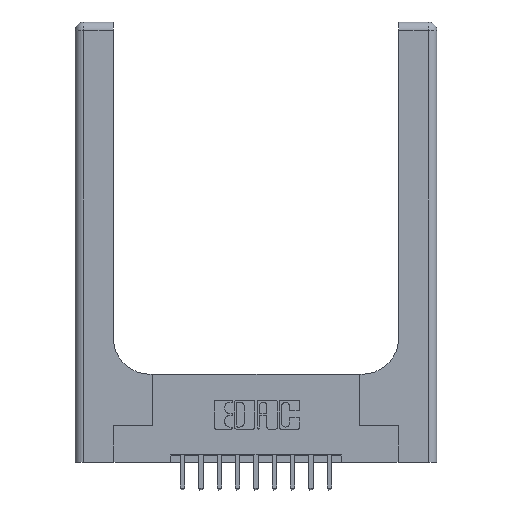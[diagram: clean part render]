
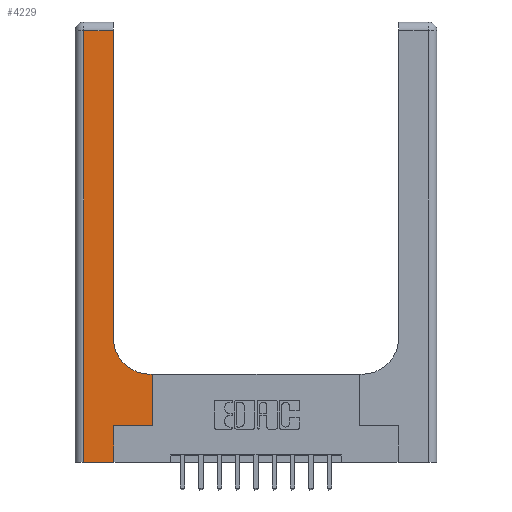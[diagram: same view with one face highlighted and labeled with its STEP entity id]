
A CAD part, top view. The second image highlights one B-rep face of the part: STEP entity #4229.
In plain terms, the highlighted planar face has unit normal (0, 0, 1).
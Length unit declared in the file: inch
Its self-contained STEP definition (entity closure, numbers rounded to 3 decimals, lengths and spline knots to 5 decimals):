
#92 = DIRECTION ( 'NONE',  ( 1., 0., 0. ) ) ;
#148 = CARTESIAN_POINT ( 'NONE',  ( 0.51, 0.85, 0.37 ) ) ;
#991 = VECTOR ( 'NONE', #5876, 39.37008 ) ;
#1242 = EDGE_CURVE ( 'NONE', #6423, #10171, #7433, .T. ) ;
#1485 = DIRECTION ( 'NONE',  ( 0., 0., -1. ) ) ;
#2095 = VERTEX_POINT ( 'NONE', #2651 ) ;
#2253 = AXIS2_PLACEMENT_3D ( 'NONE', #148, #13304, #92 ) ;
#2651 = CARTESIAN_POINT ( 'NONE',  ( 0.265, 0.25, 0.37 ) ) ;
#2841 = EDGE_CURVE ( 'NONE', #8647, #10609, #8145, .T. ) ;
#2886 = ORIENTED_EDGE ( 'NONE', *, *, #13141, .T. ) ;
#3201 = CARTESIAN_POINT ( 'NONE',  ( 0.26, 2.94, 0.37 ) ) ;
#3312 = DIRECTION ( 'NONE',  ( 0., 1., 0. ) ) ;
#3357 = DIRECTION ( 'NONE',  ( 1., 0., 0. ) ) ;
#3389 = LINE ( 'NONE', #8070, #9646 ) ;
#3525 = CARTESIAN_POINT ( 'NONE',  ( 0.528, 0.25, 0.37 ) ) ;
#3585 = ORIENTED_EDGE ( 'NONE', *, *, #7296, .T. ) ;
#3734 = CARTESIAN_POINT ( 'NONE',  ( 0.26, 0.6, 0.37 ) ) ;
#4045 = EDGE_CURVE ( 'NONE', #10171, #8647, #3389, .T. ) ;
#4153 = FACE_OUTER_BOUND ( 'NONE', #10988, .T. ) ;
#4197 = LINE ( 'NONE', #5805, #14605 ) ;
#4229 = ADVANCED_FACE ( 'NONE', ( #4153 ), #5670, .F. ) ;
#4361 = CARTESIAN_POINT ( 'NONE',  ( 0.51, 0.6, 0.37 ) ) ;
#4505 = VECTOR ( 'NONE', #3312, 39.37008 ) ;
#4637 = DIRECTION ( 'NONE',  ( 0., -1., 0. ) ) ;
#4786 = ORIENTED_EDGE ( 'NONE', *, *, #9829, .T. ) ;
#4878 = ORIENTED_EDGE ( 'NONE', *, *, #6588, .T. ) ;
#5089 = VECTOR ( 'NONE', #3357, 39.37008 ) ;
#5237 = CARTESIAN_POINT ( 'NONE',  ( 0.06, 0., 0.37 ) ) ;
#5670 = PLANE ( 'NONE',  #6874 ) ;
#5805 = CARTESIAN_POINT ( 'NONE',  ( 0.26, 3., 0.37 ) ) ;
#5876 = DIRECTION ( 'NONE',  ( -1., 0., 0. ) ) ;
#6007 = DIRECTION ( 'NONE',  ( -1., 0., 0. ) ) ;
#6138 = LINE ( 'NONE', #3525, #8016 ) ;
#6423 = VERTEX_POINT ( 'NONE', #3201 ) ;
#6440 = VERTEX_POINT ( 'NONE', #6805 ) ;
#6588 = EDGE_CURVE ( 'NONE', #2095, #15572, #8312, .T. ) ;
#6777 = LINE ( 'NONE', #13138, #4505 ) ;
#6805 = CARTESIAN_POINT ( 'NONE',  ( 0.528, 0.6, 0.37 ) ) ;
#6874 = AXIS2_PLACEMENT_3D ( 'NONE', #15600, #1485, #14887 ) ;
#7296 = EDGE_CURVE ( 'NONE', #10609, #2095, #6777, .T. ) ;
#7433 = LINE ( 'NONE', #15512, #991 ) ;
#7696 = DIRECTION ( 'NONE',  ( 1., 0., 0. ) ) ;
#7759 = VERTEX_POINT ( 'NONE', #4361 ) ;
#8016 = VECTOR ( 'NONE', #8232, 39.37008 ) ;
#8070 = CARTESIAN_POINT ( 'NONE',  ( 0.06, 3., 0.37 ) ) ;
#8143 = EDGE_CURVE ( 'NONE', #6440, #7759, #14305, .T. ) ;
#8145 = LINE ( 'NONE', #12641, #14573 ) ;
#8232 = DIRECTION ( 'NONE',  ( 0., 1., 0. ) ) ;
#8312 = LINE ( 'NONE', #13019, #5089 ) ;
#8647 = VERTEX_POINT ( 'NONE', #5237 ) ;
#9331 = CARTESIAN_POINT ( 'NONE',  ( 0.06, 2.94, 0.37 ) ) ;
#9454 = DIRECTION ( 'NONE',  ( 0., 1., 0. ) ) ;
#9646 = VECTOR ( 'NONE', #4637, 39.37008 ) ;
#9759 = EDGE_CURVE ( 'NONE', #15572, #6440, #6138, .T. ) ;
#9829 = EDGE_CURVE ( 'NONE', #7759, #13471, #10476, .T. ) ;
#10171 = VERTEX_POINT ( 'NONE', #9331 ) ;
#10476 = CIRCLE ( 'NONE', #2253, 0.25 ) ;
#10550 = ORIENTED_EDGE ( 'NONE', *, *, #9759, .T. ) ;
#10609 = VERTEX_POINT ( 'NONE', #14940 ) ;
#10988 = EDGE_LOOP ( 'NONE', ( #2886, #15451, #15349, #13473, #3585, #4878, #10550, #11073, #4786 ) ) ;
#11073 = ORIENTED_EDGE ( 'NONE', *, *, #8143, .T. ) ;
#11643 = CARTESIAN_POINT ( 'NONE',  ( 0.528, 0.25, 0.37 ) ) ;
#12407 = VECTOR ( 'NONE', #6007, 39.37008 ) ;
#12641 = CARTESIAN_POINT ( 'NONE',  ( 0., 0., 0.37 ) ) ;
#13019 = CARTESIAN_POINT ( 'NONE',  ( 0.265, 0.25, 0.37 ) ) ;
#13138 = CARTESIAN_POINT ( 'NONE',  ( 0.265, 0., 0.37 ) ) ;
#13141 = EDGE_CURVE ( 'NONE', #13471, #6423, #4197, .T. ) ;
#13304 = DIRECTION ( 'NONE',  ( 0., 0., -1. ) ) ;
#13471 = VERTEX_POINT ( 'NONE', #14136 ) ;
#13473 = ORIENTED_EDGE ( 'NONE', *, *, #2841, .T. ) ;
#14136 = CARTESIAN_POINT ( 'NONE',  ( 0.26, 0.85, 0.37 ) ) ;
#14305 = LINE ( 'NONE', #3734, #12407 ) ;
#14573 = VECTOR ( 'NONE', #7696, 39.37008 ) ;
#14605 = VECTOR ( 'NONE', #9454, 39.37008 ) ;
#14887 = DIRECTION ( 'NONE',  ( -1., 0., 0. ) ) ;
#14940 = CARTESIAN_POINT ( 'NONE',  ( 0.265, 0., 0.37 ) ) ;
#15349 = ORIENTED_EDGE ( 'NONE', *, *, #4045, .T. ) ;
#15451 = ORIENTED_EDGE ( 'NONE', *, *, #1242, .T. ) ;
#15512 = CARTESIAN_POINT ( 'NONE',  ( 0., 2.94, 0.37 ) ) ;
#15572 = VERTEX_POINT ( 'NONE', #11643 ) ;
#15600 = CARTESIAN_POINT ( 'NONE',  ( 0., 3., 0.37 ) ) ;
